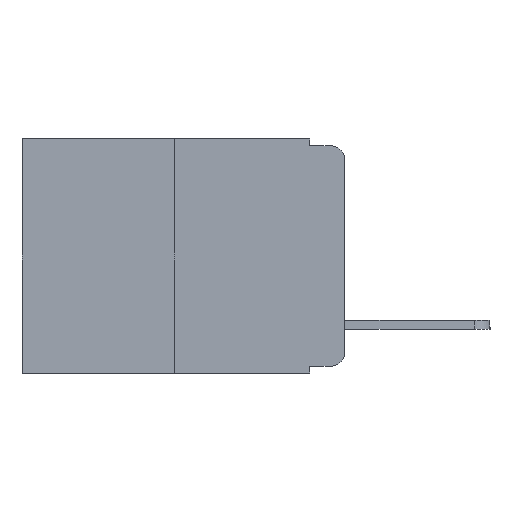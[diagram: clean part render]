
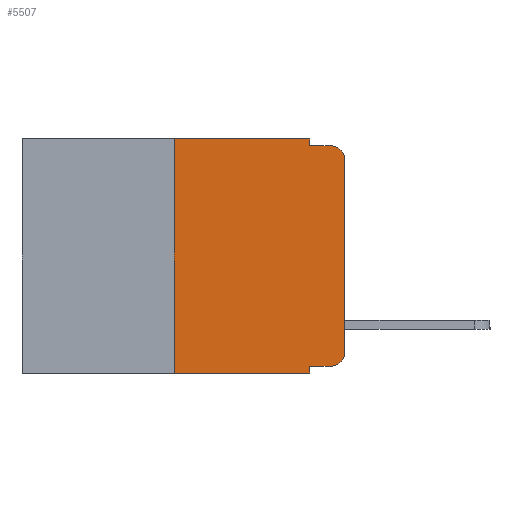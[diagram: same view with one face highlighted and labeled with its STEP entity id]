
A CAD part, left-side view. The second image highlights one B-rep face of the part: STEP entity #5507.
In plain terms, the highlighted planar face has unit normal (-1, 0, 0).
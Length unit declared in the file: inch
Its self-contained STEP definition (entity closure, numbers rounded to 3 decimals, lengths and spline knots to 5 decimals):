
#146 = VERTEX_POINT ( 'NONE', #6072 ) ;
#217 = VECTOR ( 'NONE', #7367, 39.37008 ) ;
#348 = VERTEX_POINT ( 'NONE', #12909 ) ;
#514 = LINE ( 'NONE', #2625, #12302 ) ;
#609 = ORIENTED_EDGE ( 'NONE', *, *, #9436, .T. ) ;
#663 = DIRECTION ( 'NONE',  ( 0., 0., -1. ) ) ;
#848 = CARTESIAN_POINT ( 'NONE',  ( 0., 0.051, -0.333 ) ) ;
#872 = LINE ( 'NONE', #3873, #7339 ) ;
#1238 = DIRECTION ( 'NONE',  ( 0., -1., 0. ) ) ;
#1445 = VERTEX_POINT ( 'NONE', #11297 ) ;
#1914 = CARTESIAN_POINT ( 'NONE',  ( 0., 0.473, 0. ) ) ;
#2050 = CARTESIAN_POINT ( 'NONE',  ( 0., 0.051, -0.01 ) ) ;
#2217 = EDGE_CURVE ( 'NONE', #11928, #1445, #10339, .T. ) ;
#2222 = AXIS2_PLACEMENT_3D ( 'NONE', #12825, #3871, #663 ) ;
#2564 = DIRECTION ( 'NONE',  ( 0., 0., -1. ) ) ;
#2625 = CARTESIAN_POINT ( 'NONE',  ( 0., 0.051, 0. ) ) ;
#2833 = VERTEX_POINT ( 'NONE', #8636 ) ;
#2993 = CARTESIAN_POINT ( 'NONE',  ( 0., 0.25, 0. ) ) ;
#3384 = FACE_OUTER_BOUND ( 'NONE', #7283, .T. ) ;
#3414 = ORIENTED_EDGE ( 'NONE', *, *, #3723, .F. ) ;
#3463 = VECTOR ( 'NONE', #5900, 39.37008 ) ;
#3492 = AXIS2_PLACEMENT_3D ( 'NONE', #12549, #12491, #11557 ) ;
#3517 = PLANE ( 'NONE',  #3492 ) ;
#3723 = EDGE_CURVE ( 'NONE', #11075, #9265, #872, .T. ) ;
#3871 = DIRECTION ( 'NONE',  ( -1., 0., 0. ) ) ;
#3873 = CARTESIAN_POINT ( 'NONE',  ( 0., 0.25, 0. ) ) ;
#3915 = VECTOR ( 'NONE', #1238, 39.37008 ) ;
#4018 = VERTEX_POINT ( 'NONE', #11037 ) ;
#4199 = ORIENTED_EDGE ( 'NONE', *, *, #10334, .T. ) ;
#4317 = CARTESIAN_POINT ( 'NONE',  ( 0., 0.051, 0. ) ) ;
#4327 = VERTEX_POINT ( 'NONE', #12432 ) ;
#4648 = LINE ( 'NONE', #1914, #3463 ) ;
#4815 = ORIENTED_EDGE ( 'NONE', *, *, #5325, .T. ) ;
#4861 = ORIENTED_EDGE ( 'NONE', *, *, #6087, .F. ) ;
#4907 = LINE ( 'NONE', #2050, #12288 ) ;
#5325 = EDGE_CURVE ( 'NONE', #1445, #146, #7445, .T. ) ;
#5362 = CARTESIAN_POINT ( 'NONE',  ( 0., 0., 0. ) ) ;
#5507 = ADVANCED_FACE ( 'NONE', ( #3384 ), #3517, .F. ) ;
#5692 = DIRECTION ( 'NONE',  ( -1., 0., 0. ) ) ;
#5900 = DIRECTION ( 'NONE',  ( 0., -1., 0. ) ) ;
#5928 = CARTESIAN_POINT ( 'NONE',  ( 0., 0.25, -0.343 ) ) ;
#6072 = CARTESIAN_POINT ( 'NONE',  ( 0., 0.02, -0.01 ) ) ;
#6087 = EDGE_CURVE ( 'NONE', #9265, #2833, #4648, .T. ) ;
#6146 = EDGE_CURVE ( 'NONE', #4018, #11928, #8477, .T. ) ;
#6199 = LINE ( 'NONE', #10313, #3915 ) ;
#6763 = ORIENTED_EDGE ( 'NONE', *, *, #8957, .F. ) ;
#6912 = DIRECTION ( 'NONE',  ( 0., -1., 0. ) ) ;
#7068 = DIRECTION ( 'NONE',  ( 0., -1., 0. ) ) ;
#7283 = EDGE_LOOP ( 'NONE', ( #11113, #4815, #11042, #8608, #4861, #3414, #609, #6763, #4199, #8812 ) ) ;
#7339 = VECTOR ( 'NONE', #9893, 39.37008 ) ;
#7367 = DIRECTION ( 'NONE',  ( 0., 0., 1. ) ) ;
#7445 = CIRCLE ( 'NONE', #12086, 0.02 ) ;
#7723 = EDGE_CURVE ( 'NONE', #2833, #12458, #514, .T. ) ;
#8477 = CIRCLE ( 'NONE', #2222, 0.02 ) ;
#8608 = ORIENTED_EDGE ( 'NONE', *, *, #7723, .F. ) ;
#8636 = CARTESIAN_POINT ( 'NONE',  ( 0., 0.051, 0. ) ) ;
#8812 = ORIENTED_EDGE ( 'NONE', *, *, #6146, .T. ) ;
#8957 = EDGE_CURVE ( 'NONE', #348, #4327, #12369, .T. ) ;
#9187 = CARTESIAN_POINT ( 'NONE',  ( 0., 0.051, -0.01 ) ) ;
#9265 = VERTEX_POINT ( 'NONE', #2993 ) ;
#9292 = DIRECTION ( 'NONE',  ( 0., 0., -1. ) ) ;
#9436 = EDGE_CURVE ( 'NONE', #11075, #4327, #6199, .T. ) ;
#9825 = CARTESIAN_POINT ( 'NONE',  ( 0., 0.02, -0.03 ) ) ;
#9886 = EDGE_CURVE ( 'NONE', #12458, #146, #4907, .T. ) ;
#9893 = DIRECTION ( 'NONE',  ( 0., 0., 1. ) ) ;
#10071 = LINE ( 'NONE', #848, #11370 ) ;
#10313 = CARTESIAN_POINT ( 'NONE',  ( 0., 0.473, -0.343 ) ) ;
#10334 = EDGE_CURVE ( 'NONE', #348, #4018, #10071, .T. ) ;
#10339 = LINE ( 'NONE', #5362, #217 ) ;
#10798 = VECTOR ( 'NONE', #12314, 39.37008 ) ;
#11037 = CARTESIAN_POINT ( 'NONE',  ( 0., 0.02, -0.333 ) ) ;
#11042 = ORIENTED_EDGE ( 'NONE', *, *, #9886, .F. ) ;
#11075 = VERTEX_POINT ( 'NONE', #5928 ) ;
#11113 = ORIENTED_EDGE ( 'NONE', *, *, #2217, .T. ) ;
#11297 = CARTESIAN_POINT ( 'NONE',  ( 0., 0., -0.03 ) ) ;
#11347 = CARTESIAN_POINT ( 'NONE',  ( 0., 0., -0.313 ) ) ;
#11370 = VECTOR ( 'NONE', #6912, 39.37008 ) ;
#11557 = DIRECTION ( 'NONE',  ( 0., 0., -1. ) ) ;
#11928 = VERTEX_POINT ( 'NONE', #11347 ) ;
#12086 = AXIS2_PLACEMENT_3D ( 'NONE', #9825, #5692, #2564 ) ;
#12288 = VECTOR ( 'NONE', #7068, 39.37008 ) ;
#12302 = VECTOR ( 'NONE', #9292, 39.37008 ) ;
#12314 = DIRECTION ( 'NONE',  ( 0., 0., -1. ) ) ;
#12369 = LINE ( 'NONE', #4317, #10798 ) ;
#12432 = CARTESIAN_POINT ( 'NONE',  ( 0., 0.051, -0.343 ) ) ;
#12458 = VERTEX_POINT ( 'NONE', #9187 ) ;
#12491 = DIRECTION ( 'NONE',  ( 1., 0., 0. ) ) ;
#12549 = CARTESIAN_POINT ( 'NONE',  ( 0., 0.473, 0. ) ) ;
#12825 = CARTESIAN_POINT ( 'NONE',  ( 0., 0.02, -0.313 ) ) ;
#12909 = CARTESIAN_POINT ( 'NONE',  ( 0., 0.051, -0.333 ) ) ;
